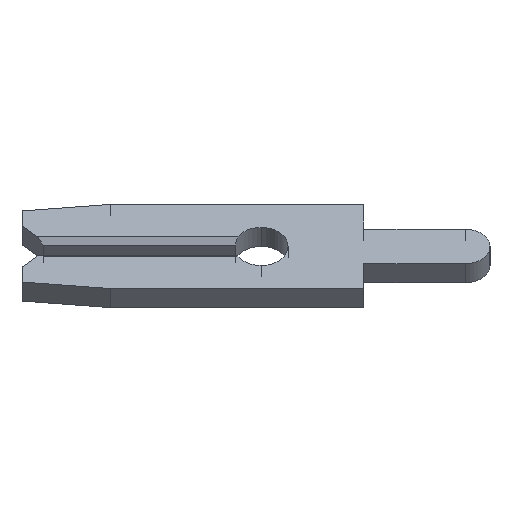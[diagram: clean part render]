
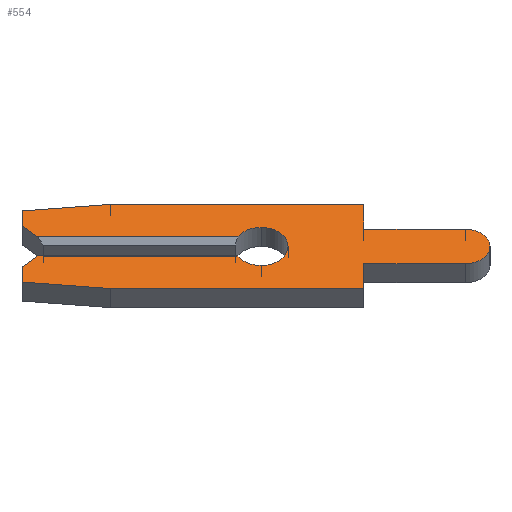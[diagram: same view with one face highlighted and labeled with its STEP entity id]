
A CAD part, left-side view. The second image highlights one B-rep face of the part: STEP entity #554.
In plain terms, the highlighted face is planar.
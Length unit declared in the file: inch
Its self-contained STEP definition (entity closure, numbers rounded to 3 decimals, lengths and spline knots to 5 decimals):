
#12 = DIRECTION ( 'NONE',  ( 0., -1., 0. ) ) ;
#19 = VERTEX_POINT ( 'NONE', #1271 ) ;
#21 = EDGE_CURVE ( 'NONE', #1257, #1232, #1079, .T. ) ;
#27 = CARTESIAN_POINT ( 'NONE',  ( -0.013, 0., 0.026 ) ) ;
#42 = ORIENTED_EDGE ( 'NONE', *, *, #745, .F. ) ;
#54 = ORIENTED_EDGE ( 'NONE', *, *, #842, .F. ) ;
#58 = CARTESIAN_POINT ( 'NONE',  ( -0.013, 0.146, -0.0575 ) ) ;
#60 = VERTEX_POINT ( 'NONE', #1688 ) ;
#85 = VECTOR ( 'NONE', #392, 39.37008 ) ;
#103 = CARTESIAN_POINT ( 'NONE',  ( -0.013, 0.146, -0.0575 ) ) ;
#104 = EDGE_CURVE ( 'NONE', #204, #608, #1593, .T. ) ;
#124 = CARTESIAN_POINT ( 'NONE',  ( -0.013, -0.099, 0.0235 ) ) ;
#126 = CARTESIAN_POINT ( 'NONE',  ( -0.013, 0.231, 0.04857 ) ) ;
#135 = LINE ( 'NONE', #126, #398 ) ;
#152 = EDGE_CURVE ( 'NONE', #1642, #19, #966, .T. ) ;
#154 = CARTESIAN_POINT ( 'NONE',  ( -0.013, -0.099, 0.0235 ) ) ;
#191 = VERTEX_POINT ( 'NONE', #1015 ) ;
#200 = CARTESIAN_POINT ( 'NONE',  ( -0.013, -0.1975, 0. ) ) ;
#204 = VERTEX_POINT ( 'NONE', #154 ) ;
#205 = CIRCLE ( 'NONE', #836, 0.026 ) ;
#219 = DIRECTION ( 'NONE',  ( 0., 1., 0. ) ) ;
#241 = EDGE_CURVE ( 'NONE', #305, #698, #778, .T. ) ;
#270 = LINE ( 'NONE', #1522, #985 ) ;
#271 = VECTOR ( 'NONE', #1809, 39.37008 ) ;
#305 = VERTEX_POINT ( 'NONE', #1836 ) ;
#313 = ORIENTED_EDGE ( 'NONE', *, *, #1710, .F. ) ;
#321 = CIRCLE ( 'NONE', #619, 0.0235 ) ;
#330 = CARTESIAN_POINT ( 'NONE',  ( -0.013, -0.1975, 0.0235 ) ) ;
#353 = EDGE_CURVE ( 'NONE', #1473, #1103, #1166, .T. ) ;
#359 = ORIENTED_EDGE ( 'NONE', *, *, #1109, .F. ) ;
#379 = LINE ( 'NONE', #103, #1006 ) ;
#392 = DIRECTION ( 'NONE',  ( 0., 0.707, 0.707 ) ) ;
#397 = EDGE_LOOP ( 'NONE', ( #1606, #914, #526, #1326, #1439, #1329, #863, #1717, #1463, #1778, #1806, #42, #988, #793, #313, #359, #54, #596 ) ) ;
#398 = VECTOR ( 'NONE', #689, 39.37008 ) ;
#427 = CARTESIAN_POINT ( 'NONE',  ( -0.013, 0.231, 0.013 ) ) ;
#438 = AXIS2_PLACEMENT_3D ( 'NONE', #1038, #1186, #590 ) ;
#445 = LINE ( 'NONE', #1623, #1561 ) ;
#470 = DIRECTION ( 'NONE',  ( 0., 0., 1. ) ) ;
#478 = CARTESIAN_POINT ( 'NONE',  ( -0.013, -0.099, -0.0235 ) ) ;
#488 = CIRCLE ( 'NONE', #937, 0.026 ) ;
#526 = ORIENTED_EDGE ( 'NONE', *, *, #241, .F. ) ;
#548 = CARTESIAN_POINT ( 'NONE',  ( -0.013, 0.216, 0.013 ) ) ;
#553 = DIRECTION ( 'NONE',  ( 0., 0.995, 0.105 ) ) ;
#554 = ADVANCED_FACE ( 'NONE', ( #1072 ), #1034, .F. ) ;
#589 = DIRECTION ( 'NONE',  ( -1., 0., 0. ) ) ;
#590 = DIRECTION ( 'NONE',  ( 0., 0., -1. ) ) ;
#596 = ORIENTED_EDGE ( 'NONE', *, *, #21, .F. ) ;
#602 = LINE ( 'NONE', #478, #1263 ) ;
#608 = VERTEX_POINT ( 'NONE', #330 ) ;
#609 = CARTESIAN_POINT ( 'NONE',  ( -0.013, 0., 0. ) ) ;
#615 = DIRECTION ( 'NONE',  ( 0., 0., 1. ) ) ;
#619 = AXIS2_PLACEMENT_3D ( 'NONE', #200, #1201, #1370 ) ;
#636 = DIRECTION ( 'NONE',  ( 0., 0., -1. ) ) ;
#658 = CARTESIAN_POINT ( 'NONE',  ( -0.013, 0.2105, 0.0075 ) ) ;
#689 = DIRECTION ( 'NONE',  ( 0., -0.995, 0.105 ) ) ;
#698 = VERTEX_POINT ( 'NONE', #27 ) ;
#715 = EDGE_CURVE ( 'NONE', #1066, #191, #602, .T. ) ;
#726 = VERTEX_POINT ( 'NONE', #769 ) ;
#745 = EDGE_CURVE ( 'NONE', #608, #1066, #321, .T. ) ;
#752 = CARTESIAN_POINT ( 'NONE',  ( -0.013, 0.02252, 0.013 ) ) ;
#767 = EDGE_CURVE ( 'NONE', #1454, #204, #1425, .T. ) ;
#769 = CARTESIAN_POINT ( 'NONE',  ( -0.013, 0.146, 0.0575 ) ) ;
#778 = CIRCLE ( 'NONE', #1112, 0.026 ) ;
#793 = ORIENTED_EDGE ( 'NONE', *, *, #767, .F. ) ;
#833 = CARTESIAN_POINT ( 'NONE',  ( -0.013, 0.216, -0.013 ) ) ;
#836 = AXIS2_PLACEMENT_3D ( 'NONE', #609, #589, #1184 ) ;
#842 = EDGE_CURVE ( 'NONE', #1232, #1033, #270, .T. ) ;
#863 = ORIENTED_EDGE ( 'NONE', *, *, #1558, .F. ) ;
#891 = LINE ( 'NONE', #1417, #1162 ) ;
#904 = DIRECTION ( 'NONE',  ( 0., -1., 0. ) ) ;
#909 = CARTESIAN_POINT ( 'NONE',  ( -0.013, -0.099, -0.0575 ) ) ;
#914 = ORIENTED_EDGE ( 'NONE', *, *, #1418, .F. ) ;
#937 = AXIS2_PLACEMENT_3D ( 'NONE', #1465, #1616, #1773 ) ;
#951 = DIRECTION ( 'NONE',  ( 0., -1., 0. ) ) ;
#966 = LINE ( 'NONE', #990, #1701 ) ;
#985 = VECTOR ( 'NONE', #615, 39.37008 ) ;
#987 = LINE ( 'NONE', #1196, #271 ) ;
#988 = ORIENTED_EDGE ( 'NONE', *, *, #104, .F. ) ;
#990 = CARTESIAN_POINT ( 'NONE',  ( -0.013, 0.231, -0.04857 ) ) ;
#1006 = VECTOR ( 'NONE', #1110, 39.37008 ) ;
#1015 = CARTESIAN_POINT ( 'NONE',  ( -0.013, -0.099, -0.0235 ) ) ;
#1026 = EDGE_CURVE ( 'NONE', #191, #1719, #891, .T. ) ;
#1033 = VERTEX_POINT ( 'NONE', #1666 ) ;
#1034 = PLANE ( 'NONE',  #438 ) ;
#1038 = CARTESIAN_POINT ( 'NONE',  ( -0.013, 0., 0. ) ) ;
#1065 = VECTOR ( 'NONE', #951, 39.37008 ) ;
#1066 = VERTEX_POINT ( 'NONE', #1812 ) ;
#1067 = CARTESIAN_POINT ( 'NONE',  ( -0.013, -0.099, 0.0575 ) ) ;
#1072 = FACE_OUTER_BOUND ( 'NONE', #397, .T. ) ;
#1079 = LINE ( 'NONE', #658, #85 ) ;
#1094 = LINE ( 'NONE', #427, #1307 ) ;
#1099 = EDGE_CURVE ( 'NONE', #1719, #1642, #379, .T. ) ;
#1103 = VERTEX_POINT ( 'NONE', #833 ) ;
#1109 = EDGE_CURVE ( 'NONE', #1033, #726, #135, .T. ) ;
#1110 = DIRECTION ( 'NONE',  ( 0., 1., 0. ) ) ;
#1112 = AXIS2_PLACEMENT_3D ( 'NONE', #1443, #1742, #1297 ) ;
#1115 = DIRECTION ( 'NONE',  ( 0., 0., -1. ) ) ;
#1120 = VECTOR ( 'NONE', #636, 39.37008 ) ;
#1151 = CARTESIAN_POINT ( 'NONE',  ( -0.013, 0.2105, -0.0075 ) ) ;
#1162 = VECTOR ( 'NONE', #1115, 39.37008 ) ;
#1166 = LINE ( 'NONE', #1151, #1789 ) ;
#1180 = CARTESIAN_POINT ( 'NONE',  ( -0.013, 0., -0.013 ) ) ;
#1184 = DIRECTION ( 'NONE',  ( 0., 0., -1. ) ) ;
#1186 = DIRECTION ( 'NONE',  ( 1., 0., 0. ) ) ;
#1188 = LINE ( 'NONE', #1180, #1655 ) ;
#1196 = CARTESIAN_POINT ( 'NONE',  ( -0.013, 0.146, 0.0575 ) ) ;
#1201 = DIRECTION ( 'NONE',  ( 1., 0., 0. ) ) ;
#1232 = VERTEX_POINT ( 'NONE', #1599 ) ;
#1257 = VERTEX_POINT ( 'NONE', #548 ) ;
#1263 = VECTOR ( 'NONE', #219, 39.37008 ) ;
#1271 = CARTESIAN_POINT ( 'NONE',  ( -0.013, 0.231, -0.04857 ) ) ;
#1297 = DIRECTION ( 'NONE',  ( 0., 0., -1. ) ) ;
#1300 = DIRECTION ( 'NONE',  ( 0., -0.707, 0.707 ) ) ;
#1307 = VECTOR ( 'NONE', #12, 39.37008 ) ;
#1326 = ORIENTED_EDGE ( 'NONE', *, *, #1426, .F. ) ;
#1329 = ORIENTED_EDGE ( 'NONE', *, *, #353, .F. ) ;
#1336 = CARTESIAN_POINT ( 'NONE',  ( -0.013, 0.231, -0.028 ) ) ;
#1342 = EDGE_CURVE ( 'NONE', #1257, #1546, #1094, .T. ) ;
#1370 = DIRECTION ( 'NONE',  ( 0., 0., 1. ) ) ;
#1374 = CARTESIAN_POINT ( 'NONE',  ( -0.013, -0.099, 0.0575 ) ) ;
#1416 = EDGE_CURVE ( 'NONE', #1103, #60, #1188, .T. ) ;
#1417 = CARTESIAN_POINT ( 'NONE',  ( -0.013, -0.099, -0.0575 ) ) ;
#1418 = EDGE_CURVE ( 'NONE', #698, #1546, #205, .T. ) ;
#1425 = LINE ( 'NONE', #1374, #1120 ) ;
#1426 = EDGE_CURVE ( 'NONE', #60, #305, #488, .T. ) ;
#1439 = ORIENTED_EDGE ( 'NONE', *, *, #1416, .F. ) ;
#1443 = CARTESIAN_POINT ( 'NONE',  ( -0.013, 0., 0. ) ) ;
#1454 = VERTEX_POINT ( 'NONE', #1067 ) ;
#1463 = ORIENTED_EDGE ( 'NONE', *, *, #1099, .F. ) ;
#1465 = CARTESIAN_POINT ( 'NONE',  ( -0.013, 0., 0. ) ) ;
#1473 = VERTEX_POINT ( 'NONE', #1336 ) ;
#1522 = CARTESIAN_POINT ( 'NONE',  ( -0.013, 0.231, 0.028 ) ) ;
#1546 = VERTEX_POINT ( 'NONE', #752 ) ;
#1558 = EDGE_CURVE ( 'NONE', #19, #1473, #445, .T. ) ;
#1561 = VECTOR ( 'NONE', #470, 39.37008 ) ;
#1593 = LINE ( 'NONE', #124, #1065 ) ;
#1599 = CARTESIAN_POINT ( 'NONE',  ( -0.013, 0.231, 0.028 ) ) ;
#1606 = ORIENTED_EDGE ( 'NONE', *, *, #1342, .T. ) ;
#1616 = DIRECTION ( 'NONE',  ( -1., 0., 0. ) ) ;
#1623 = CARTESIAN_POINT ( 'NONE',  ( -0.013, 0.231, -0.028 ) ) ;
#1642 = VERTEX_POINT ( 'NONE', #58 ) ;
#1655 = VECTOR ( 'NONE', #904, 39.37008 ) ;
#1666 = CARTESIAN_POINT ( 'NONE',  ( -0.013, 0.231, 0.04857 ) ) ;
#1688 = CARTESIAN_POINT ( 'NONE',  ( -0.013, 0.02252, -0.013 ) ) ;
#1701 = VECTOR ( 'NONE', #553, 39.37008 ) ;
#1710 = EDGE_CURVE ( 'NONE', #726, #1454, #987, .T. ) ;
#1717 = ORIENTED_EDGE ( 'NONE', *, *, #152, .F. ) ;
#1719 = VERTEX_POINT ( 'NONE', #909 ) ;
#1742 = DIRECTION ( 'NONE',  ( -1., 0., 0. ) ) ;
#1773 = DIRECTION ( 'NONE',  ( 0., 0., -1. ) ) ;
#1778 = ORIENTED_EDGE ( 'NONE', *, *, #1026, .F. ) ;
#1789 = VECTOR ( 'NONE', #1300, 39.37008 ) ;
#1806 = ORIENTED_EDGE ( 'NONE', *, *, #715, .F. ) ;
#1809 = DIRECTION ( 'NONE',  ( 0., -1., 0. ) ) ;
#1812 = CARTESIAN_POINT ( 'NONE',  ( -0.013, -0.1975, -0.0235 ) ) ;
#1836 = CARTESIAN_POINT ( 'NONE',  ( -0.013, 0., -0.026 ) ) ;
